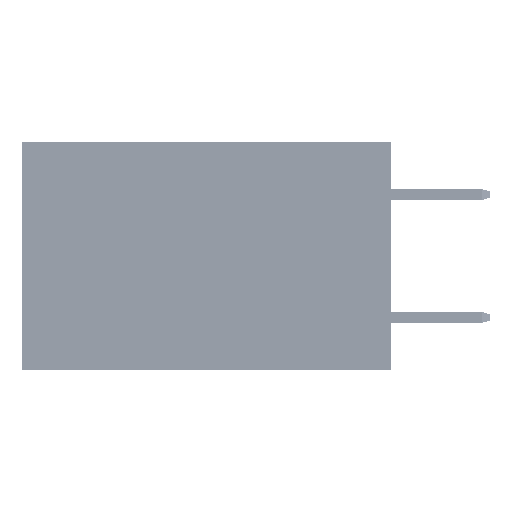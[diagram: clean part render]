
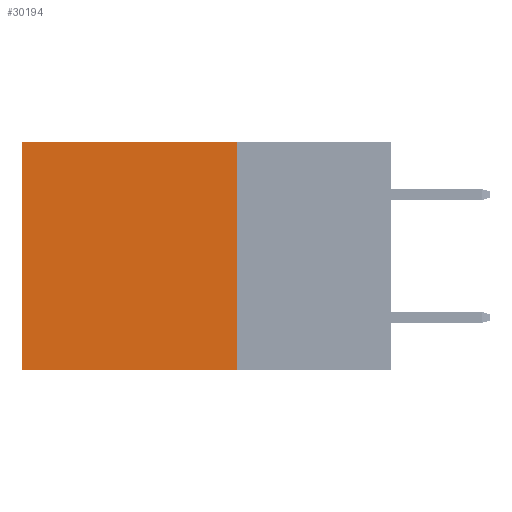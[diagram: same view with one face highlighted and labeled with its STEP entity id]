
A CAD part, left-side view. The second image highlights one B-rep face of the part: STEP entity #30194.
In plain terms, the highlighted planar face has unit normal (-1, 0, 0).
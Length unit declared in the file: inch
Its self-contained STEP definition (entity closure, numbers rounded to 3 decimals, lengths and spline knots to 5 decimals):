
#864 = LINE ( 'NONE', #24232, #10915 ) ;
#2152 = LINE ( 'NONE', #48231, #40423 ) ;
#2422 = LINE ( 'NONE', #33356, #31950 ) ;
#7805 = CARTESIAN_POINT ( 'NONE',  ( 0.2875, 0.25, 0. ) ) ;
#8409 = AXIS2_PLACEMENT_3D ( 'NONE', #13030, #43514, #28145 ) ;
#8985 = CARTESIAN_POINT ( 'NONE',  ( 0.2875, 0.6, 0. ) ) ;
#10915 = VECTOR ( 'NONE', #23507, 39.37008 ) ;
#11799 = VERTEX_POINT ( 'NONE', #43048 ) ;
#13030 = CARTESIAN_POINT ( 'NONE',  ( 0.2875, 0.25, 0. ) ) ;
#13593 = ORIENTED_EDGE ( 'NONE', *, *, #47893, .F. ) ;
#16064 = CARTESIAN_POINT ( 'NONE',  ( 0.2875, 0.25, 0. ) ) ;
#17849 = EDGE_CURVE ( 'NONE', #34418, #23370, #35205, .T. ) ;
#19591 = DIRECTION ( 'NONE',  ( 0., 1., 0. ) ) ;
#20206 = ORIENTED_EDGE ( 'NONE', *, *, #34603, .T. ) ;
#23370 = VERTEX_POINT ( 'NONE', #8985 ) ;
#23507 = DIRECTION ( 'NONE',  ( 0., 0., -1. ) ) ;
#23564 = EDGE_CURVE ( 'NONE', #27402, #11799, #2152, .T. ) ;
#24232 = CARTESIAN_POINT ( 'NONE',  ( 0.2875, 0.25, 0. ) ) ;
#25552 = DIRECTION ( 'NONE',  ( 0., 1., 0. ) ) ;
#27402 = VERTEX_POINT ( 'NONE', #46782 ) ;
#28145 = DIRECTION ( 'NONE',  ( 0., 0., -1. ) ) ;
#30194 = ADVANCED_FACE ( 'NONE', ( #35945 ), #32917, .F. ) ;
#31312 = EDGE_LOOP ( 'NONE', ( #20206, #47561, #13593, #46363 ) ) ;
#31950 = VECTOR ( 'NONE', #37142, 39.37008 ) ;
#32917 = PLANE ( 'NONE',  #8409 ) ;
#33356 = CARTESIAN_POINT ( 'NONE',  ( 0.2875, 0.6, 0. ) ) ;
#34418 = VERTEX_POINT ( 'NONE', #7805 ) ;
#34603 = EDGE_CURVE ( 'NONE', #23370, #11799, #2422, .T. ) ;
#35205 = LINE ( 'NONE', #16064, #35890 ) ;
#35890 = VECTOR ( 'NONE', #19591, 39.37008 ) ;
#35945 = FACE_OUTER_BOUND ( 'NONE', #31312, .T. ) ;
#37142 = DIRECTION ( 'NONE',  ( 0., 0., -1. ) ) ;
#40423 = VECTOR ( 'NONE', #25552, 39.37008 ) ;
#43048 = CARTESIAN_POINT ( 'NONE',  ( 0.2875, 0.6, -0.37 ) ) ;
#43514 = DIRECTION ( 'NONE',  ( 1., 0., 0. ) ) ;
#46363 = ORIENTED_EDGE ( 'NONE', *, *, #17849, .T. ) ;
#46782 = CARTESIAN_POINT ( 'NONE',  ( 0.2875, 0.25, -0.37 ) ) ;
#47561 = ORIENTED_EDGE ( 'NONE', *, *, #23564, .F. ) ;
#47893 = EDGE_CURVE ( 'NONE', #34418, #27402, #864, .T. ) ;
#48231 = CARTESIAN_POINT ( 'NONE',  ( 0.2875, 0.25, -0.37 ) ) ;
